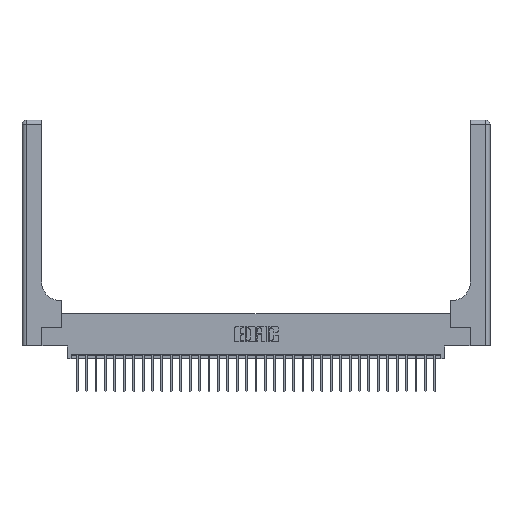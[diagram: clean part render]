
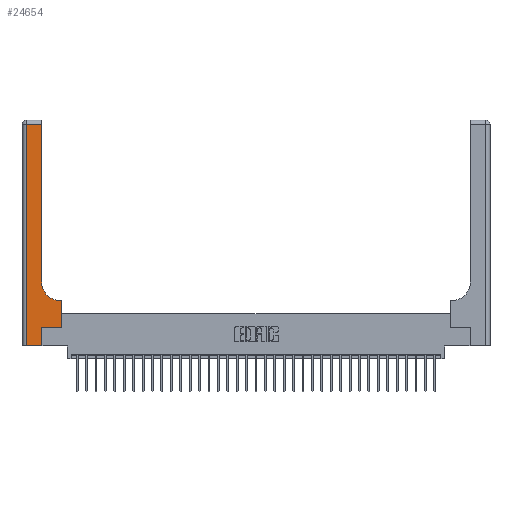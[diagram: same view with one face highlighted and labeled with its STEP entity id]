
A CAD part, top view. The second image highlights one B-rep face of the part: STEP entity #24654.
In plain terms, the highlighted planar face has unit normal (0, 0, 1).
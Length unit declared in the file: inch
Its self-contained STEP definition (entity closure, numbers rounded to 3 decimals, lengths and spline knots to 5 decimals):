
#113 = CARTESIAN_POINT ( 'NONE',  ( 0.26, 0.6, 0.37 ) ) ;
#308 = VECTOR ( 'NONE', #10042, 39.37008 ) ;
#421 = VECTOR ( 'NONE', #27951, 39.37008 ) ;
#1616 = DIRECTION ( 'NONE',  ( 0., 0., -1. ) ) ;
#1790 = LINE ( 'NONE', #9335, #6999 ) ;
#2811 = LINE ( 'NONE', #12744, #308 ) ;
#3346 = CARTESIAN_POINT ( 'NONE',  ( 0.265, 0., 0.37 ) ) ;
#3547 = VERTEX_POINT ( 'NONE', #16390 ) ;
#4036 = ORIENTED_EDGE ( 'NONE', *, *, #12719, .T. ) ;
#4146 = VERTEX_POINT ( 'NONE', #7195 ) ;
#4624 = EDGE_CURVE ( 'NONE', #17513, #8134, #2811, .T. ) ;
#4805 = DIRECTION ( 'NONE',  ( -1., 0., 0. ) ) ;
#5824 = DIRECTION ( 'NONE',  ( 0., 1., 0. ) ) ;
#6115 = ORIENTED_EDGE ( 'NONE', *, *, #26850, .T. ) ;
#6491 = CARTESIAN_POINT ( 'NONE',  ( 0., 0., 0.37 ) ) ;
#6999 = VECTOR ( 'NONE', #26474, 39.37008 ) ;
#7195 = CARTESIAN_POINT ( 'NONE',  ( 0.265, 0.25, 0.37 ) ) ;
#7200 = CARTESIAN_POINT ( 'NONE',  ( 0., 3., 0.37 ) ) ;
#8078 = EDGE_CURVE ( 'NONE', #23431, #8962, #22497, .T. ) ;
#8134 = VERTEX_POINT ( 'NONE', #22344 ) ;
#8275 = VECTOR ( 'NONE', #5824, 39.37008 ) ;
#8551 = LINE ( 'NONE', #30164, #8275 ) ;
#8676 = DIRECTION ( 'NONE',  ( 1., 0., 0. ) ) ;
#8962 = VERTEX_POINT ( 'NONE', #28449 ) ;
#9335 = CARTESIAN_POINT ( 'NONE',  ( 0.265, 0.25, 0.37 ) ) ;
#9378 = ORIENTED_EDGE ( 'NONE', *, *, #4624, .T. ) ;
#9439 = CIRCLE ( 'NONE', #12486, 0.25 ) ;
#9450 = ORIENTED_EDGE ( 'NONE', *, *, #13983, .T. ) ;
#9496 = VERTEX_POINT ( 'NONE', #27926 ) ;
#9901 = DIRECTION ( 'NONE',  ( -1., 0., 0. ) ) ;
#10042 = DIRECTION ( 'NONE',  ( -1., 0., 0. ) ) ;
#10654 = LINE ( 'NONE', #18039, #421 ) ;
#11213 = ORIENTED_EDGE ( 'NONE', *, *, #17899, .T. ) ;
#11298 = LINE ( 'NONE', #6491, #16302 ) ;
#11703 = DIRECTION ( 'NONE',  ( 0., 0., -1. ) ) ;
#12023 = CARTESIAN_POINT ( 'NONE',  ( 0.06, 0., 0.37 ) ) ;
#12393 = ORIENTED_EDGE ( 'NONE', *, *, #21744, .T. ) ;
#12486 = AXIS2_PLACEMENT_3D ( 'NONE', #21179, #1616, #8676 ) ;
#12719 = EDGE_CURVE ( 'NONE', #9496, #4146, #25143, .T. ) ;
#12744 = CARTESIAN_POINT ( 'NONE',  ( 0., 2.94, 0.37 ) ) ;
#13525 = VERTEX_POINT ( 'NONE', #12023 ) ;
#13983 = EDGE_CURVE ( 'NONE', #8962, #19019, #15169, .T. ) ;
#15169 = LINE ( 'NONE', #113, #16490 ) ;
#16093 = CARTESIAN_POINT ( 'NONE',  ( 0.26, 2.94, 0.37 ) ) ;
#16118 = DIRECTION ( 'NONE',  ( 1., 0., 0. ) ) ;
#16302 = VECTOR ( 'NONE', #16118, 39.37008 ) ;
#16390 = CARTESIAN_POINT ( 'NONE',  ( 0.26, 0.85, 0.37 ) ) ;
#16490 = VECTOR ( 'NONE', #9901, 39.37008 ) ;
#16834 = PLANE ( 'NONE',  #29292 ) ;
#17513 = VERTEX_POINT ( 'NONE', #16093 ) ;
#17514 = ORIENTED_EDGE ( 'NONE', *, *, #18057, .T. ) ;
#17899 = EDGE_CURVE ( 'NONE', #8134, #13525, #10654, .T. ) ;
#17942 = VECTOR ( 'NONE', #17943, 39.37008 ) ;
#17943 = DIRECTION ( 'NONE',  ( 0., 1., 0. ) ) ;
#18039 = CARTESIAN_POINT ( 'NONE',  ( 0.06, 3., 0.37 ) ) ;
#18057 = EDGE_CURVE ( 'NONE', #13525, #9496, #11298, .T. ) ;
#19019 = VERTEX_POINT ( 'NONE', #21164 ) ;
#19394 = VECTOR ( 'NONE', #24753, 39.37008 ) ;
#21164 = CARTESIAN_POINT ( 'NONE',  ( 0.51, 0.6, 0.37 ) ) ;
#21179 = CARTESIAN_POINT ( 'NONE',  ( 0.51, 0.85, 0.37 ) ) ;
#21744 = EDGE_CURVE ( 'NONE', #3547, #17513, #8551, .T. ) ;
#22344 = CARTESIAN_POINT ( 'NONE',  ( 0.06, 2.94, 0.37 ) ) ;
#22497 = LINE ( 'NONE', #26845, #19394 ) ;
#23431 = VERTEX_POINT ( 'NONE', #27793 ) ;
#24654 = ADVANCED_FACE ( 'NONE', ( #28667 ), #16834, .F. ) ;
#24753 = DIRECTION ( 'NONE',  ( 0., 1., 0. ) ) ;
#25143 = LINE ( 'NONE', #3346, #17942 ) ;
#25271 = ORIENTED_EDGE ( 'NONE', *, *, #8078, .T. ) ;
#26474 = DIRECTION ( 'NONE',  ( 1., 0., 0. ) ) ;
#26845 = CARTESIAN_POINT ( 'NONE',  ( 0.528, 0.25, 0.37 ) ) ;
#26850 = EDGE_CURVE ( 'NONE', #19019, #3547, #9439, .T. ) ;
#27793 = CARTESIAN_POINT ( 'NONE',  ( 0.528, 0.25, 0.37 ) ) ;
#27926 = CARTESIAN_POINT ( 'NONE',  ( 0.265, 0., 0.37 ) ) ;
#27951 = DIRECTION ( 'NONE',  ( 0., -1., 0. ) ) ;
#27981 = EDGE_LOOP ( 'NONE', ( #12393, #9378, #11213, #17514, #4036, #30255, #25271, #9450, #6115 ) ) ;
#28449 = CARTESIAN_POINT ( 'NONE',  ( 0.528, 0.6, 0.37 ) ) ;
#28667 = FACE_OUTER_BOUND ( 'NONE', #27981, .T. ) ;
#29254 = EDGE_CURVE ( 'NONE', #4146, #23431, #1790, .T. ) ;
#29292 = AXIS2_PLACEMENT_3D ( 'NONE', #7200, #11703, #4805 ) ;
#30164 = CARTESIAN_POINT ( 'NONE',  ( 0.26, 3., 0.37 ) ) ;
#30255 = ORIENTED_EDGE ( 'NONE', *, *, #29254, .T. ) ;
